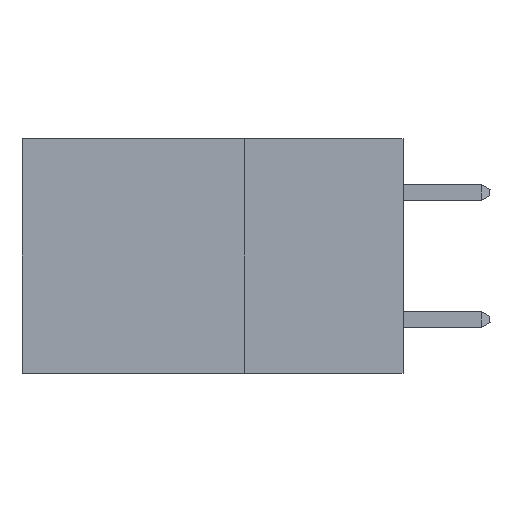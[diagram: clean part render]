
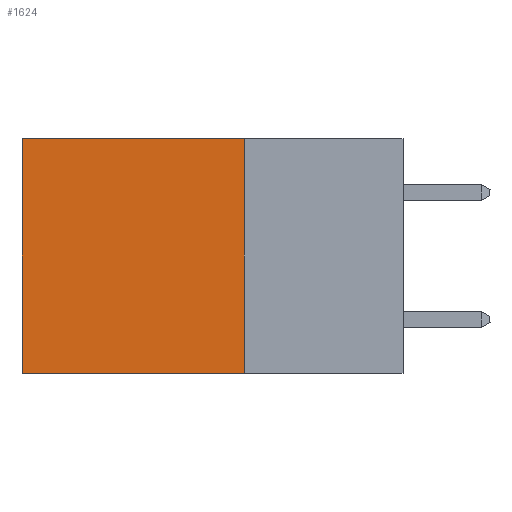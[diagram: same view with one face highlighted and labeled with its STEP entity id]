
A CAD part, left-side view. The second image highlights one B-rep face of the part: STEP entity #1624.
In plain terms, the highlighted planar face has unit normal (-1, 0, 0).
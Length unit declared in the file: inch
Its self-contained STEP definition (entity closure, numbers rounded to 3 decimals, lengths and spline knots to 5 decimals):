
#1624 = ADVANCED_FACE ( 'NONE', ( #28421 ), #5626, .F. ) ;
#2137 = VECTOR ( 'NONE', #15710, 39.37008 ) ;
#3275 = ORIENTED_EDGE ( 'NONE', *, *, #26947, .T. ) ;
#3894 = VERTEX_POINT ( 'NONE', #25173 ) ;
#5041 = EDGE_CURVE ( 'NONE', #16384, #13495, #17455, .T. ) ;
#5626 = PLANE ( 'NONE',  #8762 ) ;
#6120 = DIRECTION ( 'NONE',  ( 0., 0., -1. ) ) ;
#6258 = ORIENTED_EDGE ( 'NONE', *, *, #5041, .T. ) ;
#7659 = CARTESIAN_POINT ( 'NONE',  ( 0.2875, 0.25, -0.37 ) ) ;
#7919 = DIRECTION ( 'NONE',  ( 1., 0., 0. ) ) ;
#8762 = AXIS2_PLACEMENT_3D ( 'NONE', #16371, #7919, #26407 ) ;
#9318 = EDGE_LOOP ( 'NONE', ( #3275, #17658, #27305, #6258 ) ) ;
#11247 = VECTOR ( 'NONE', #6120, 39.37008 ) ;
#11642 = LINE ( 'NONE', #24242, #11247 ) ;
#11809 = VECTOR ( 'NONE', #29303, 39.37008 ) ;
#12735 = EDGE_CURVE ( 'NONE', #15893, #3894, #25888, .T. ) ;
#13495 = VERTEX_POINT ( 'NONE', #32738 ) ;
#15430 = EDGE_CURVE ( 'NONE', #16384, #15893, #11642, .T. ) ;
#15710 = DIRECTION ( 'NONE',  ( 0., 1., 0. ) ) ;
#15893 = VERTEX_POINT ( 'NONE', #7659 ) ;
#16120 = CARTESIAN_POINT ( 'NONE',  ( 0.2875, 0.25, 0. ) ) ;
#16371 = CARTESIAN_POINT ( 'NONE',  ( 0.2875, 0.25, 0. ) ) ;
#16384 = VERTEX_POINT ( 'NONE', #16120 ) ;
#17455 = LINE ( 'NONE', #23430, #2137 ) ;
#17658 = ORIENTED_EDGE ( 'NONE', *, *, #12735, .F. ) ;
#19043 = LINE ( 'NONE', #33430, #19857 ) ;
#19857 = VECTOR ( 'NONE', #20644, 39.37008 ) ;
#20644 = DIRECTION ( 'NONE',  ( 0., 0., -1. ) ) ;
#23430 = CARTESIAN_POINT ( 'NONE',  ( 0.2875, 0.25, 0. ) ) ;
#24242 = CARTESIAN_POINT ( 'NONE',  ( 0.2875, 0.25, 0. ) ) ;
#25173 = CARTESIAN_POINT ( 'NONE',  ( 0.2875, 0.6, -0.37 ) ) ;
#25888 = LINE ( 'NONE', #31486, #11809 ) ;
#26407 = DIRECTION ( 'NONE',  ( 0., 0., -1. ) ) ;
#26947 = EDGE_CURVE ( 'NONE', #13495, #3894, #19043, .T. ) ;
#27305 = ORIENTED_EDGE ( 'NONE', *, *, #15430, .F. ) ;
#28421 = FACE_OUTER_BOUND ( 'NONE', #9318, .T. ) ;
#29303 = DIRECTION ( 'NONE',  ( 0., 1., 0. ) ) ;
#31486 = CARTESIAN_POINT ( 'NONE',  ( 0.2875, 0.25, -0.37 ) ) ;
#32738 = CARTESIAN_POINT ( 'NONE',  ( 0.2875, 0.6, 0. ) ) ;
#33430 = CARTESIAN_POINT ( 'NONE',  ( 0.2875, 0.6, 0. ) ) ;
